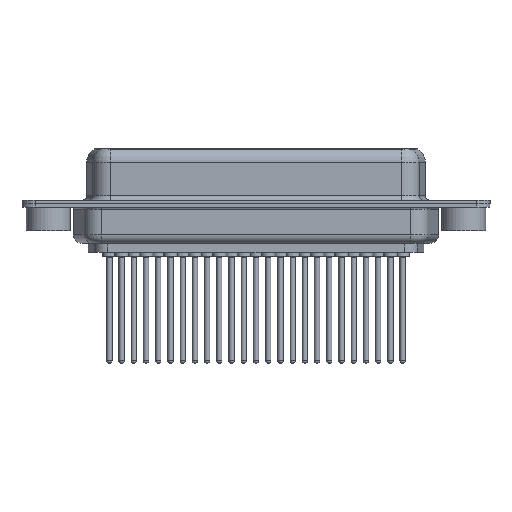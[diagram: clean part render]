
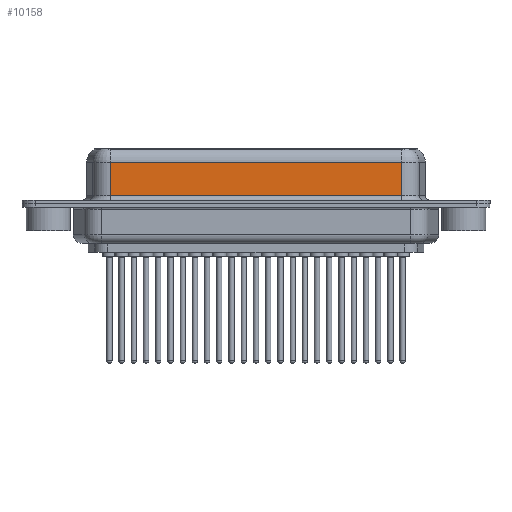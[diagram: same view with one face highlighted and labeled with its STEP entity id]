
A CAD part, front view. The second image highlights one B-rep face of the part: STEP entity #10158.
In plain terms, the highlighted planar face has unit normal (0, -1, 0).
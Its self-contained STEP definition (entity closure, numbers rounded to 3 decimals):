
#1251 = VECTOR ( 'NONE', #20192, 1000. ) ;
#1351 = DIRECTION ( 'NONE',  ( 1., 0., 0. ) ) ;
#1601 = ORIENTED_EDGE ( 'NONE', *, *, #6004, .T. ) ;
#1909 = DIRECTION ( 'NONE',  ( -1., 0., 0. ) ) ;
#1996 = DIRECTION ( 'NONE',  ( 0., 1., 0. ) ) ;
#2786 = VERTEX_POINT ( 'NONE', #12817 ) ;
#3117 = LINE ( 'NONE', #17936, #5449 ) ;
#3214 = FACE_OUTER_BOUND ( 'NONE', #20707, .T. ) ;
#3322 = CARTESIAN_POINT ( 'NONE',  ( 40.037, -3.95, 6.4 ) ) ;
#4238 = ORIENTED_EDGE ( 'NONE', *, *, #17899, .T. ) ;
#4399 = VERTEX_POINT ( 'NONE', #12365 ) ;
#5189 = PLANE ( 'NONE',  #5272 ) ;
#5272 = AXIS2_PLACEMENT_3D ( 'NONE', #3322, #1996, #21755 ) ;
#5449 = VECTOR ( 'NONE', #1351, 1000. ) ;
#5616 = LINE ( 'NONE', #15304, #15219 ) ;
#6004 = EDGE_CURVE ( 'NONE', #13460, #2786, #18534, .T. ) ;
#6834 = CARTESIAN_POINT ( 'NONE',  ( 7.013, -3.95, 4.65 ) ) ;
#8910 = CARTESIAN_POINT ( 'NONE',  ( 40.037, -3.95, 0.9 ) ) ;
#10008 = CARTESIAN_POINT ( 'NONE',  ( 7.013, -3.95, 6.4 ) ) ;
#10158 = ADVANCED_FACE ( 'NONE', ( #3214 ), #5189, .F. ) ;
#11804 = ORIENTED_EDGE ( 'NONE', *, *, #15162, .F. ) ;
#12144 = CARTESIAN_POINT ( 'NONE',  ( 40.037, -3.95, 4.65 ) ) ;
#12365 = CARTESIAN_POINT ( 'NONE',  ( 40.037, -3.95, 4.65 ) ) ;
#12817 = CARTESIAN_POINT ( 'NONE',  ( 7.013, -3.95, 0.9 ) ) ;
#13460 = VERTEX_POINT ( 'NONE', #6834 ) ;
#15162 = EDGE_CURVE ( 'NONE', #4399, #16965, #5616, .T. ) ;
#15219 = VECTOR ( 'NONE', #20644, 1000. ) ;
#15304 = CARTESIAN_POINT ( 'NONE',  ( 40.037, -3.95, 6.4 ) ) ;
#16265 = EDGE_CURVE ( 'NONE', #2786, #16965, #3117, .T. ) ;
#16721 = ORIENTED_EDGE ( 'NONE', *, *, #16265, .T. ) ;
#16965 = VERTEX_POINT ( 'NONE', #8910 ) ;
#17511 = VECTOR ( 'NONE', #1909, 1000. ) ;
#17899 = EDGE_CURVE ( 'NONE', #4399, #13460, #18591, .T. ) ;
#17936 = CARTESIAN_POINT ( 'NONE',  ( 40.037, -3.95, 0.9 ) ) ;
#18534 = LINE ( 'NONE', #10008, #1251 ) ;
#18591 = LINE ( 'NONE', #12144, #17511 ) ;
#20192 = DIRECTION ( 'NONE',  ( 0., 0., -1. ) ) ;
#20644 = DIRECTION ( 'NONE',  ( 0., 0., -1. ) ) ;
#20707 = EDGE_LOOP ( 'NONE', ( #11804, #4238, #1601, #16721 ) ) ;
#21755 = DIRECTION ( 'NONE',  ( 0., 0., 1. ) ) ;
